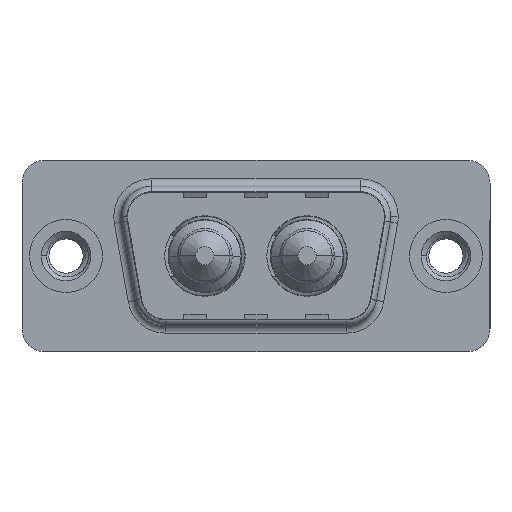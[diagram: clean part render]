
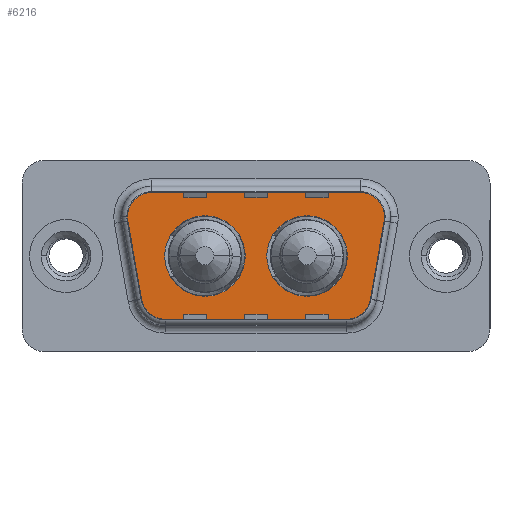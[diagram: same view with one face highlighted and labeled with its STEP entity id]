
A CAD part, top view. The second image highlights one B-rep face of the part: STEP entity #6216.
In plain terms, the highlighted planar face has unit normal (0, 0, 1).
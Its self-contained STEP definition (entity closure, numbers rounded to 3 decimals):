
#102 = VERTEX_POINT ( 'NONE', #2959 ) ;
#575 = VERTEX_POINT ( 'NONE', #8177 ) ;
#584 = AXIS2_PLACEMENT_3D ( 'NONE', #8909, #3507, #9825 ) ;
#609 = VECTOR ( 'NONE', #7139, 1000. ) ;
#630 = CARTESIAN_POINT ( 'NONE',  ( 19.564, 2.9, 0. ) ) ;
#775 = EDGE_CURVE ( 'NONE', #2961, #4098, #7920, .T. ) ;
#855 = EDGE_CURVE ( 'NONE', #4042, #2961, #9466, .T. ) ;
#872 = CIRCLE ( 'NONE', #8436, 2. ) ;
#873 = CIRCLE ( 'NONE', #6889, 2.65 ) ;
#906 = DIRECTION ( 'NONE',  ( 0., 0., 1. ) ) ;
#924 = ORIENTED_EDGE ( 'NONE', *, *, #8121, .T. ) ;
#1034 = CIRCLE ( 'NONE', #6404, 2.65 ) ;
#1416 = DIRECTION ( 'NONE',  ( -1., 0., 0. ) ) ;
#1424 = DIRECTION ( 'NONE',  ( 1., 0., 0. ) ) ;
#1570 = CARTESIAN_POINT ( 'NONE',  ( 3.466, 2.553, 0. ) ) ;
#1590 = EDGE_CURVE ( 'NONE', #11305, #1917, #2893, .T. ) ;
#1684 = DIRECTION ( 'NONE',  ( 0., 0., 1. ) ) ;
#1803 = CARTESIAN_POINT ( 'NONE',  ( 21.564, 2.9, 0. ) ) ;
#1917 = VERTEX_POINT ( 'NONE', #5751 ) ;
#2295 = VERTEX_POINT ( 'NONE', #10394 ) ;
#2356 = AXIS2_PLACEMENT_3D ( 'NONE', #3847, #10170, #4759 ) ;
#2730 = EDGE_LOOP ( 'NONE', ( #4742, #7799 ) ) ;
#2893 = CIRCLE ( 'NONE', #7105, 2. ) ;
#2959 = CARTESIAN_POINT ( 'NONE',  ( 6.49, 0., 0. ) ) ;
#2961 = VERTEX_POINT ( 'NONE', #7571 ) ;
#3012 = DIRECTION ( 'NONE',  ( 0., 0., 1. ) ) ;
#3029 = LINE ( 'NONE', #9815, #609 ) ;
#3035 = EDGE_CURVE ( 'NONE', #575, #11450, #872, .T. ) ;
#3497 = CIRCLE ( 'NONE', #9546, 2. ) ;
#3507 = DIRECTION ( 'NONE',  ( 0., 0., 1. ) ) ;
#3625 = CARTESIAN_POINT ( 'NONE',  ( 11.79, 0., 0. ) ) ;
#3691 = ORIENTED_EDGE ( 'NONE', *, *, #3035, .T. ) ;
#3847 = CARTESIAN_POINT ( 'NONE',  ( 9.14, 0., 0. ) ) ;
#3856 = FACE_BOUND ( 'NONE', #5084, .T. ) ;
#4004 = DIRECTION ( 'NONE',  ( 0., 0., 1. ) ) ;
#4042 = VERTEX_POINT ( 'NONE', #10635 ) ;
#4098 = VERTEX_POINT ( 'NONE', #5939 ) ;
#4147 = CARTESIAN_POINT ( 'NONE',  ( 19.564, 2.9, 0. ) ) ;
#4157 = AXIS2_PLACEMENT_3D ( 'NONE', #9844, #906, #4945 ) ;
#4170 = LINE ( 'NONE', #1570, #6566 ) ;
#4375 = ORIENTED_EDGE ( 'NONE', *, *, #855, .T. ) ;
#4517 = EDGE_CURVE ( 'NONE', #11450, #10516, #4170, .T. ) ;
#4550 = DIRECTION ( 'NONE',  ( 1., 0., 0. ) ) ;
#4633 = CARTESIAN_POINT ( 'NONE',  ( 5.436, 2.9, 0. ) ) ;
#4651 = EDGE_CURVE ( 'NONE', #4098, #7677, #3029, .T. ) ;
#4742 = ORIENTED_EDGE ( 'NONE', *, *, #6260, .F. ) ;
#4759 = DIRECTION ( 'NONE',  ( 1., 0., 0. ) ) ;
#4796 = DIRECTION ( 'NONE',  ( -1., 0., 0. ) ) ;
#4836 = ORIENTED_EDGE ( 'NONE', *, *, #11091, .T. ) ;
#4865 = ORIENTED_EDGE ( 'NONE', *, *, #4651, .T. ) ;
#4945 = DIRECTION ( 'NONE',  ( 1., 0., 0. ) ) ;
#5056 = DIRECTION ( 'NONE',  ( -1., 0., 0. ) ) ;
#5072 = AXIS2_PLACEMENT_3D ( 'NONE', #11331, #6826, #1424 ) ;
#5084 = EDGE_LOOP ( 'NONE', ( #9506, #9289 ) ) ;
#5094 = DIRECTION ( 'NONE',  ( 0., 0., 1. ) ) ;
#5165 = DIRECTION ( 'NONE',  ( 0.174, -0.985, 0. ) ) ;
#5290 = ORIENTED_EDGE ( 'NONE', *, *, #775, .T. ) ;
#5493 = EDGE_CURVE ( 'NONE', #2295, #5552, #1034, .T. ) ;
#5552 = VERTEX_POINT ( 'NONE', #8461 ) ;
#5751 = CARTESIAN_POINT ( 'NONE',  ( 19.564, 4.9, 0. ) ) ;
#5939 = CARTESIAN_POINT ( 'NONE',  ( 20.511, -3.247, 0. ) ) ;
#5983 = FACE_BOUND ( 'NONE', #2730, .T. ) ;
#6216 = ADVANCED_FACE ( 'NONE', ( #3856, #5983, #10785 ), #7715, .T. ) ;
#6260 = EDGE_CURVE ( 'NONE', #11631, #102, #873, .T. ) ;
#6389 = CIRCLE ( 'NONE', #584, 2.65 ) ;
#6404 = AXIS2_PLACEMENT_3D ( 'NONE', #8420, #3012, #9319 ) ;
#6472 = EDGE_CURVE ( 'NONE', #5552, #2295, #6389, .T. ) ;
#6566 = VECTOR ( 'NONE', #5165, 1000. ) ;
#6728 = ORIENTED_EDGE ( 'NONE', *, *, #1590, .T. ) ;
#6801 = ORIENTED_EDGE ( 'NONE', *, *, #8289, .T. ) ;
#6826 = DIRECTION ( 'NONE',  ( 0., 0., 1. ) ) ;
#6889 = AXIS2_PLACEMENT_3D ( 'NONE', #10511, #5094, #11406 ) ;
#6933 = DIRECTION ( 'NONE',  ( 0., 0., 1. ) ) ;
#7076 = VECTOR ( 'NONE', #4550, 1000. ) ;
#7095 = CARTESIAN_POINT ( 'NONE',  ( 6.459, -2.9, 0. ) ) ;
#7105 = AXIS2_PLACEMENT_3D ( 'NONE', #630, #6933, #4796 ) ;
#7139 = DIRECTION ( 'NONE',  ( 0.174, 0.985, 0. ) ) ;
#7171 = CARTESIAN_POINT ( 'NONE',  ( 21.534, 2.553, 0. ) ) ;
#7196 = CIRCLE ( 'NONE', #2356, 2.65 ) ;
#7324 = EDGE_CURVE ( 'NONE', #102, #11631, #7196, .T. ) ;
#7571 = CARTESIAN_POINT ( 'NONE',  ( 18.541, -4.9, 0. ) ) ;
#7677 = VERTEX_POINT ( 'NONE', #7171 ) ;
#7715 = PLANE ( 'NONE',  #5072 ) ;
#7752 = ORIENTED_EDGE ( 'NONE', *, *, #4517, .T. ) ;
#7799 = ORIENTED_EDGE ( 'NONE', *, *, #7324, .F. ) ;
#7920 = CIRCLE ( 'NONE', #4157, 2. ) ;
#7999 = DIRECTION ( 'NONE',  ( -1., 0., 0. ) ) ;
#8121 = EDGE_CURVE ( 'NONE', #1917, #575, #9141, .T. ) ;
#8177 = CARTESIAN_POINT ( 'NONE',  ( 5.436, 4.9, 0. ) ) ;
#8232 = DIRECTION ( 'NONE',  ( 1., 0., 0. ) ) ;
#8289 = EDGE_CURVE ( 'NONE', #10516, #4042, #3497, .T. ) ;
#8339 = CARTESIAN_POINT ( 'NONE',  ( 6.459, -4.9, 0. ) ) ;
#8420 = CARTESIAN_POINT ( 'NONE',  ( 15.86, 0., 0. ) ) ;
#8436 = AXIS2_PLACEMENT_3D ( 'NONE', #4633, #4004, #8232 ) ;
#8461 = CARTESIAN_POINT ( 'NONE',  ( 13.21, 0., 0. ) ) ;
#8909 = CARTESIAN_POINT ( 'NONE',  ( 15.86, 0., 0. ) ) ;
#9027 = EDGE_LOOP ( 'NONE', ( #5290, #4865, #4836, #6728, #924, #3691, #7752, #6801, #4375 ) ) ;
#9141 = LINE ( 'NONE', #10464, #11542 ) ;
#9171 = AXIS2_PLACEMENT_3D ( 'NONE', #4147, #10467, #5056 ) ;
#9289 = ORIENTED_EDGE ( 'NONE', *, *, #6472, .F. ) ;
#9319 = DIRECTION ( 'NONE',  ( 1., 0., 0. ) ) ;
#9466 = LINE ( 'NONE', #8339, #7076 ) ;
#9506 = ORIENTED_EDGE ( 'NONE', *, *, #5493, .F. ) ;
#9546 = AXIS2_PLACEMENT_3D ( 'NONE', #7095, #1684, #7999 ) ;
#9815 = CARTESIAN_POINT ( 'NONE',  ( 21.534, 2.553, 0. ) ) ;
#9825 = DIRECTION ( 'NONE',  ( 1., 0., 0. ) ) ;
#9844 = CARTESIAN_POINT ( 'NONE',  ( 18.541, -2.9, 0. ) ) ;
#10170 = DIRECTION ( 'NONE',  ( 0., 0., 1. ) ) ;
#10335 = CIRCLE ( 'NONE', #9171, 2. ) ;
#10394 = CARTESIAN_POINT ( 'NONE',  ( 18.51, 0., 0. ) ) ;
#10464 = CARTESIAN_POINT ( 'NONE',  ( 5.436, 4.9, 0. ) ) ;
#10467 = DIRECTION ( 'NONE',  ( 0., 0., 1. ) ) ;
#10511 = CARTESIAN_POINT ( 'NONE',  ( 9.14, 0., 0. ) ) ;
#10516 = VERTEX_POINT ( 'NONE', #11480 ) ;
#10635 = CARTESIAN_POINT ( 'NONE',  ( 6.459, -4.9, 0. ) ) ;
#10785 = FACE_OUTER_BOUND ( 'NONE', #9027, .T. ) ;
#11076 = CARTESIAN_POINT ( 'NONE',  ( 3.466, 2.553, 0. ) ) ;
#11091 = EDGE_CURVE ( 'NONE', #7677, #11305, #10335, .T. ) ;
#11305 = VERTEX_POINT ( 'NONE', #1803 ) ;
#11331 = CARTESIAN_POINT ( 'NONE',  ( 18.541, -2.9, 0. ) ) ;
#11406 = DIRECTION ( 'NONE',  ( 1., 0., 0. ) ) ;
#11450 = VERTEX_POINT ( 'NONE', #11076 ) ;
#11480 = CARTESIAN_POINT ( 'NONE',  ( 4.489, -3.247, 0. ) ) ;
#11542 = VECTOR ( 'NONE', #1416, 1000. ) ;
#11631 = VERTEX_POINT ( 'NONE', #3625 ) ;
